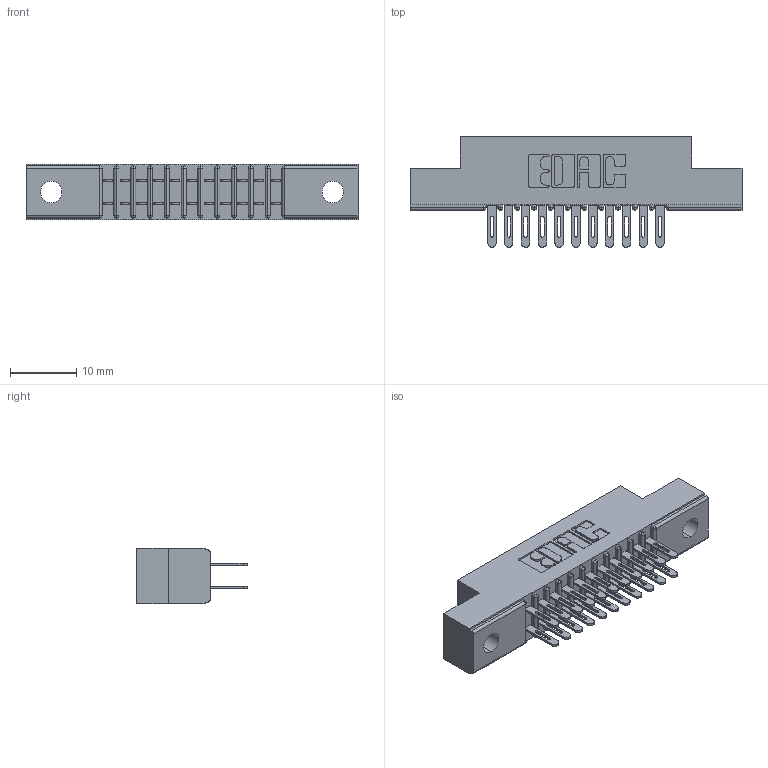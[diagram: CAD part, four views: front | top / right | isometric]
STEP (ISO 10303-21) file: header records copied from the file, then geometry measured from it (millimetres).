
FILE_DESCRIPTION (( 'STEP AP203' ), '1' );
FILE_NAME ('341-022-500-202.STEP', '2018-08-06T17:13:08', ( '' ), ( '' ), 'SwSTEP 2.0', 'SolidWorks 2016', '' );
FILE_SCHEMA (( 'CONFIG_CONTROL_DESIGN' ));
Length unit declared in the file: inch
Products named in the file (3): 341 Part_.128 (3.25) Dia Mounting Holes; 341-292-001_341-292-100; 341-022-500-202
Assembly tree (23 placements, depth 2):
  341-022-500-202
    341 Part_.128 (3.25) Dia Mounting Holes
    341-292-001_341-292-100  x22
Bounding box: 50.16 x 16.69 x 8.38 mm (x, y, z)
Volume: 2874.2 mm3; surface area: 5245.4 mm2
Topology: 23 solids, 23 shells, 1568 faces, 4529 edges, 2934 vertices
Faces by surface type: plane 904, cylinder 620, sphere 24, torus 20
Entity records: 17452 total; most frequent: CARTESIAN_POINT 2901, ORIENTED_EDGE 2878, DIRECTION 2841, EDGE_CURVE 1439, VECTOR 1125, LINE 1125, VERTEX_POINT 918, AXIS2_PLACEMENT_3D 858
